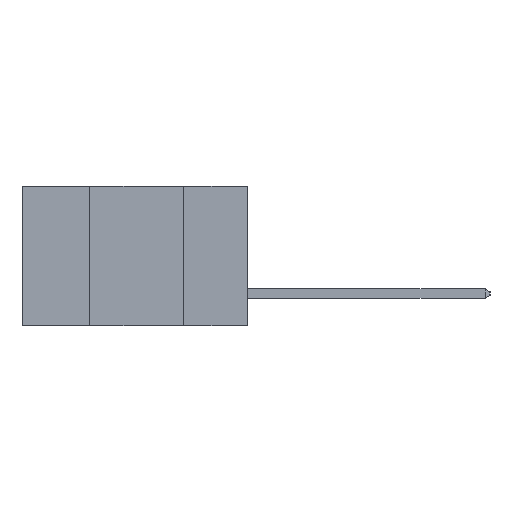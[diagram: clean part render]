
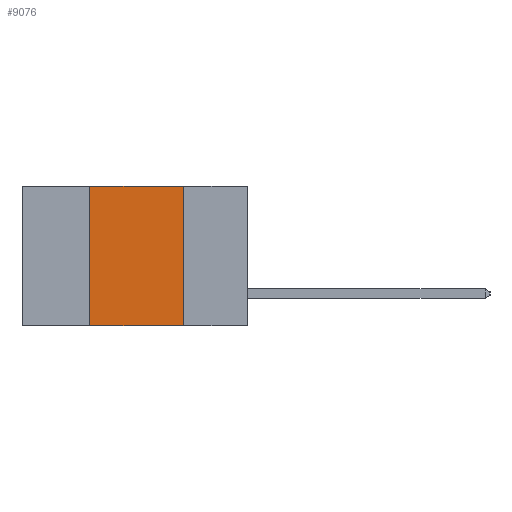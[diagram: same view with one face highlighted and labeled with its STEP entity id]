
A CAD part, left-side view. The second image highlights one B-rep face of the part: STEP entity #9076.
In plain terms, the highlighted planar face has unit normal (-1, 0, 0).
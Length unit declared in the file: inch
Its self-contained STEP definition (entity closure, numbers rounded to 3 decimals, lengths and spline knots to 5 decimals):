
#107 = VERTEX_POINT ( 'NONE', #2349 ) ;
#499 = FACE_OUTER_BOUND ( 'NONE', #4182, .T. ) ;
#528 = ORIENTED_EDGE ( 'NONE', *, *, #1149, .F. ) ;
#661 = ORIENTED_EDGE ( 'NONE', *, *, #8540, .F. ) ;
#666 = CARTESIAN_POINT ( 'NONE',  ( 0., 0.17, -0.37 ) ) ;
#704 = ORIENTED_EDGE ( 'NONE', *, *, #4236, .F. ) ;
#914 = VECTOR ( 'NONE', #3359, 39.37008 ) ;
#1149 = EDGE_CURVE ( 'NONE', #6191, #8844, #1765, .T. ) ;
#1467 = ORIENTED_EDGE ( 'NONE', *, *, #7198, .T. ) ;
#1685 = CARTESIAN_POINT ( 'NONE',  ( 0., 0.17, 0. ) ) ;
#1765 = LINE ( 'NONE', #666, #3766 ) ;
#1876 = LINE ( 'NONE', #3503, #7948 ) ;
#1897 = CARTESIAN_POINT ( 'NONE',  ( 0., 0.17, -0.37 ) ) ;
#2349 = CARTESIAN_POINT ( 'NONE',  ( 0., 0.42, 0. ) ) ;
#2402 = VERTEX_POINT ( 'NONE', #10283 ) ;
#3113 = CARTESIAN_POINT ( 'NONE',  ( 0., 0.6, 0. ) ) ;
#3223 = CARTESIAN_POINT ( 'NONE',  ( 0., 0.6, 0. ) ) ;
#3359 = DIRECTION ( 'NONE',  ( 0., -1., 0. ) ) ;
#3503 = CARTESIAN_POINT ( 'NONE',  ( 0., 0.42, -0.37 ) ) ;
#3766 = VECTOR ( 'NONE', #6613, 39.37008 ) ;
#4182 = EDGE_LOOP ( 'NONE', ( #528, #661, #704, #1467 ) ) ;
#4236 = EDGE_CURVE ( 'NONE', #2402, #107, #1876, .T. ) ;
#4347 = DIRECTION ( 'NONE',  ( 0., 0., 1. ) ) ;
#4647 = LINE ( 'NONE', #3223, #8863 ) ;
#5602 = DIRECTION ( 'NONE',  ( 0., 0., -1. ) ) ;
#6191 = VERTEX_POINT ( 'NONE', #1685 ) ;
#6613 = DIRECTION ( 'NONE',  ( 0., 0., -1. ) ) ;
#7198 = EDGE_CURVE ( 'NONE', #2402, #8844, #9618, .T. ) ;
#7317 = DIRECTION ( 'NONE',  ( 0., -1., 0. ) ) ;
#7457 = CARTESIAN_POINT ( 'NONE',  ( 0., 0.6, -0.37 ) ) ;
#7948 = VECTOR ( 'NONE', #4347, 39.37008 ) ;
#8540 = EDGE_CURVE ( 'NONE', #107, #6191, #4647, .T. ) ;
#8844 = VERTEX_POINT ( 'NONE', #1897 ) ;
#8863 = VECTOR ( 'NONE', #7317, 39.37008 ) ;
#9076 = ADVANCED_FACE ( 'NONE', ( #499 ), #10259, .F. ) ;
#9618 = LINE ( 'NONE', #7457, #914 ) ;
#9960 = AXIS2_PLACEMENT_3D ( 'NONE', #3113, #10287, #5602 ) ;
#10259 = PLANE ( 'NONE',  #9960 ) ;
#10283 = CARTESIAN_POINT ( 'NONE',  ( 0., 0.42, -0.37 ) ) ;
#10287 = DIRECTION ( 'NONE',  ( 1., 0., 0. ) ) ;
